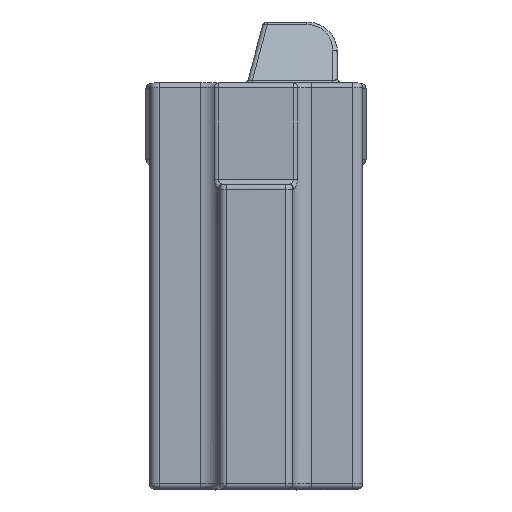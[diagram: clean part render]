
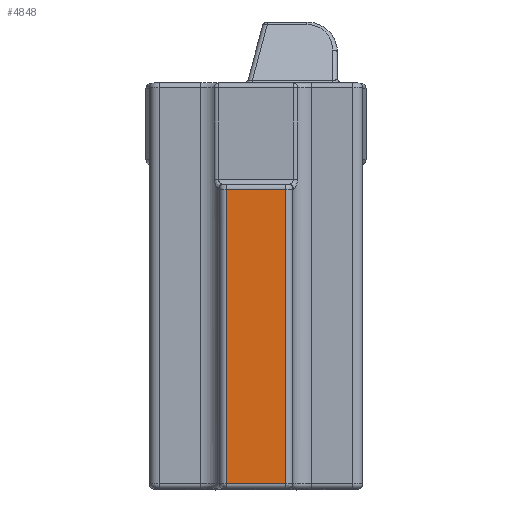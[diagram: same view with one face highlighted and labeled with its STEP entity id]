
A CAD part, top view. The second image highlights one B-rep face of the part: STEP entity #4848.
In plain terms, the highlighted planar face has unit normal (0, 0, 1).
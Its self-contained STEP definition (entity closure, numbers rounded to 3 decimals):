
#166=PLANE('',#5422);
#367=LINE('',#9654,#625);
#419=LINE('',#13360,#677);
#446=LINE('',#13781,#704);
#447=LINE('',#13782,#705);
#625=VECTOR('',#6111,1000.);
#677=VECTOR('',#6543,1000.);
#704=VECTOR('',#6736,1000.);
#705=VECTOR('',#6737,1000.);
#1102=FACE_OUTER_BOUND('',#1412,.T.);
#1412=EDGE_LOOP('',(#4294,#4295,#4296,#4297));
#2178=VERTEX_POINT('',#9646);
#2181=VERTEX_POINT('',#9652);
#2290=VERTEX_POINT('',#13355);
#2291=VERTEX_POINT('',#13359);
#2713=EDGE_CURVE('',#2178,#2181,#367,.T.);
#2933=EDGE_CURVE('',#2290,#2291,#419,.T.);
#3007=EDGE_CURVE('',#2181,#2290,#446,.T.);
#3008=EDGE_CURVE('',#2291,#2178,#447,.T.);
#4294=ORIENTED_EDGE('',*,*,#3007,.T.);
#4295=ORIENTED_EDGE('',*,*,#2933,.T.);
#4296=ORIENTED_EDGE('',*,*,#3008,.T.);
#4297=ORIENTED_EDGE('',*,*,#2713,.T.);
#4848=ADVANCED_FACE('',(#1102),#166,.T.);
#5422=AXIS2_PLACEMENT_3D('',#13780,#6734,#6735);
#6111=DIRECTION('',(-1.,0.,0.));
#6543=DIRECTION('',(1.,0.,0.));
#6734=DIRECTION('center_axis',(0.,0.,
1.));
#6735=DIRECTION('ref_axis',(0.,-1.,0.));
#6736=DIRECTION('',(0.,-1.,0.));
#6737=DIRECTION('',(0.,1.,0.));
#9646=CARTESIAN_POINT('',(2.324,-126.057,57.277));
#9652=CARTESIAN_POINT('',(-2.324,-126.057,57.277));
#9654=CARTESIAN_POINT('',(0.,-126.057,57.277));
#13355=CARTESIAN_POINT('',(-2.324,-149.12,57.277));
#13359=CARTESIAN_POINT('',(2.324,-149.12,57.277));
#13360=CARTESIAN_POINT('',(0.,-149.12,57.277));
#13780=CARTESIAN_POINT('Origin',(-2.324,-126.057,57.277));
#13781=CARTESIAN_POINT('',(-2.324,-137.589,57.277));
#13782=CARTESIAN_POINT('',(2.324,-137.589,57.277));
